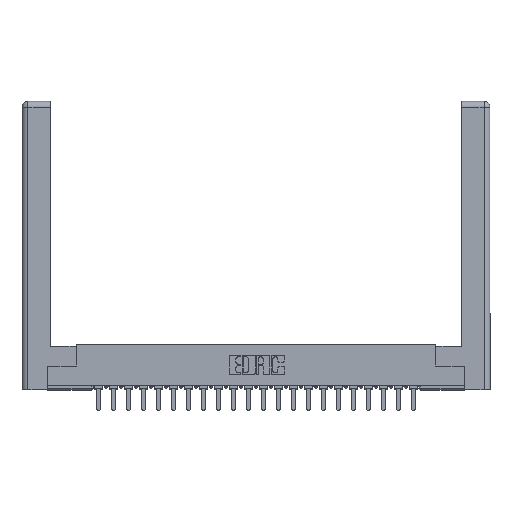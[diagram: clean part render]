
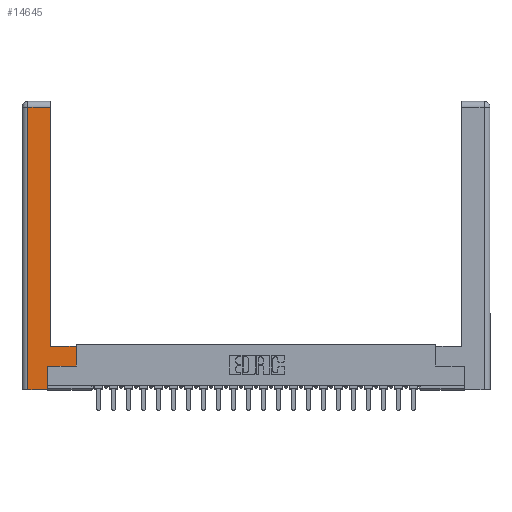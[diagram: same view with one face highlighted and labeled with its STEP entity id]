
A CAD part, top view. The second image highlights one B-rep face of the part: STEP entity #14645.
In plain terms, the highlighted planar face has unit normal (0, 0, 1).
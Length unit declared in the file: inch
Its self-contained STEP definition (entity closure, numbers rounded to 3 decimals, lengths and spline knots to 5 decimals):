
#944 = EDGE_CURVE ( 'NONE', #7150, #3121, #3639, .T. ) ;
#1295 = DIRECTION ( 'NONE',  ( 1., 0., 0. ) ) ;
#1370 = VECTOR ( 'NONE', #4972, 39.37008 ) ;
#1842 = VERTEX_POINT ( 'NONE', #12348 ) ;
#2493 = EDGE_CURVE ( 'NONE', #23967, #9515, #11288, .T. ) ;
#2745 = CARTESIAN_POINT ( 'NONE',  ( 0.265, 0., 0. ) ) ;
#2949 = DIRECTION ( 'NONE',  ( 0., 0., -1. ) ) ;
#3121 = VERTEX_POINT ( 'NONE', #14290 ) ;
#3639 = LINE ( 'NONE', #13820, #19412 ) ;
#4117 = VECTOR ( 'NONE', #14094, 39.37008 ) ;
#4661 = ORIENTED_EDGE ( 'NONE', *, *, #16963, .T. ) ;
#4696 = CARTESIAN_POINT ( 'NONE',  ( 0.565, 0.45, 0. ) ) ;
#4740 = VECTOR ( 'NONE', #21979, 39.37008 ) ;
#4972 = DIRECTION ( 'NONE',  ( 0., 1., 0. ) ) ;
#7046 = CARTESIAN_POINT ( 'NONE',  ( 0.265, 0.245, 0. ) ) ;
#7150 = VERTEX_POINT ( 'NONE', #20266 ) ;
#7322 = CARTESIAN_POINT ( 'NONE',  ( 0.0615, 0., 0. ) ) ;
#7451 = EDGE_CURVE ( 'NONE', #3121, #24200, #23717, .T. ) ;
#7458 = EDGE_CURVE ( 'NONE', #24200, #23967, #14783, .T. ) ;
#7554 = LINE ( 'NONE', #22269, #20958 ) ;
#8280 = LINE ( 'NONE', #8318, #17824 ) ;
#8318 = CARTESIAN_POINT ( 'NONE',  ( 0.295, 0.45, 0. ) ) ;
#8479 = DIRECTION ( 'NONE',  ( -1., 0., 0. ) ) ;
#9055 = EDGE_CURVE ( 'NONE', #1842, #11818, #7554, .T. ) ;
#9515 = VERTEX_POINT ( 'NONE', #2745 ) ;
#9792 = ORIENTED_EDGE ( 'NONE', *, *, #17599, .T. ) ;
#10552 = CARTESIAN_POINT ( 'NONE',  ( 0.265, 0., 0. ) ) ;
#10581 = DIRECTION ( 'NONE',  ( -1., 0., 0. ) ) ;
#11058 = ORIENTED_EDGE ( 'NONE', *, *, #2493, .T. ) ;
#11288 = LINE ( 'NONE', #10552, #4740 ) ;
#11818 = VERTEX_POINT ( 'NONE', #13022 ) ;
#12290 = ORIENTED_EDGE ( 'NONE', *, *, #944, .T. ) ;
#12314 = EDGE_CURVE ( 'NONE', #9515, #1842, #22237, .T. ) ;
#12348 = CARTESIAN_POINT ( 'NONE',  ( 0.265, 0.245, 0. ) ) ;
#12386 = ORIENTED_EDGE ( 'NONE', *, *, #7458, .T. ) ;
#13022 = CARTESIAN_POINT ( 'NONE',  ( 0.565, 0.245, 0. ) ) ;
#13466 = ORIENTED_EDGE ( 'NONE', *, *, #7451, .T. ) ;
#13581 = VECTOR ( 'NONE', #24396, 39.37008 ) ;
#13820 = CARTESIAN_POINT ( 'NONE',  ( 0.295, 3., 0. ) ) ;
#14094 = DIRECTION ( 'NONE',  ( 0., 1., 0. ) ) ;
#14290 = CARTESIAN_POINT ( 'NONE',  ( 0.295, 2.94, 0. ) ) ;
#14645 = ADVANCED_FACE ( 'NONE', ( #15530 ), #24082, .F. ) ;
#14783 = LINE ( 'NONE', #7322, #13581 ) ;
#15302 = CARTESIAN_POINT ( 'NONE',  ( 0.0615, 2.94, 0. ) ) ;
#15530 = FACE_OUTER_BOUND ( 'NONE', #18612, .T. ) ;
#16021 = ORIENTED_EDGE ( 'NONE', *, *, #9055, .T. ) ;
#16333 = LINE ( 'NONE', #17956, #4117 ) ;
#16922 = CARTESIAN_POINT ( 'NONE',  ( 0.0615, 2.94, 0. ) ) ;
#16963 = EDGE_CURVE ( 'NONE', #21965, #7150, #8280, .T. ) ;
#17599 = EDGE_CURVE ( 'NONE', #11818, #21965, #16333, .T. ) ;
#17824 = VECTOR ( 'NONE', #8479, 39.37008 ) ;
#17956 = CARTESIAN_POINT ( 'NONE',  ( 0.565, 0.45, 0. ) ) ;
#18072 = AXIS2_PLACEMENT_3D ( 'NONE', #22188, #2949, #10581 ) ;
#18612 = EDGE_LOOP ( 'NONE', ( #12290, #13466, #12386, #11058, #18637, #16021, #9792, #4661 ) ) ;
#18637 = ORIENTED_EDGE ( 'NONE', *, *, #12314, .T. ) ;
#18659 = VECTOR ( 'NONE', #24313, 39.37008 ) ;
#19412 = VECTOR ( 'NONE', #21256, 39.37008 ) ;
#20266 = CARTESIAN_POINT ( 'NONE',  ( 0.295, 0.45, 0. ) ) ;
#20958 = VECTOR ( 'NONE', #1295, 39.37008 ) ;
#21256 = DIRECTION ( 'NONE',  ( 0., 1., 0. ) ) ;
#21965 = VERTEX_POINT ( 'NONE', #4696 ) ;
#21979 = DIRECTION ( 'NONE',  ( 1., 0., 0. ) ) ;
#22188 = CARTESIAN_POINT ( 'NONE',  ( 0., 0., 0. ) ) ;
#22237 = LINE ( 'NONE', #7046, #1370 ) ;
#22269 = CARTESIAN_POINT ( 'NONE',  ( 0.565, 0.245, 0. ) ) ;
#23717 = LINE ( 'NONE', #16922, #18659 ) ;
#23889 = CARTESIAN_POINT ( 'NONE',  ( 0.0615, 0., 0. ) ) ;
#23967 = VERTEX_POINT ( 'NONE', #23889 ) ;
#24082 = PLANE ( 'NONE',  #18072 ) ;
#24200 = VERTEX_POINT ( 'NONE', #15302 ) ;
#24313 = DIRECTION ( 'NONE',  ( -1., 0., 0. ) ) ;
#24396 = DIRECTION ( 'NONE',  ( 0., -1., 0. ) ) ;
